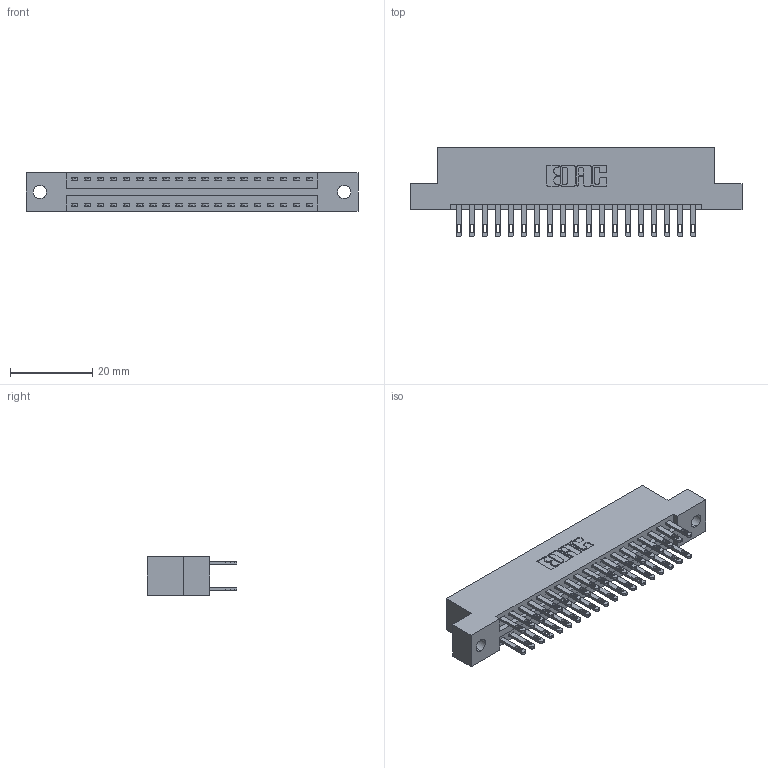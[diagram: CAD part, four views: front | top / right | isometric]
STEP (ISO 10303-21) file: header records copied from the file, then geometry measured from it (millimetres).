
FILE_DESCRIPTION (( 'STEP AP203' ), '1' );
FILE_NAME ('896-038-500-202.STEP', '2021-07-27T20:37:14', ( '' ), ( '' ), 'SwSTEP 2.0', 'SolidWorks 2020', '' );
FILE_SCHEMA (( 'CONFIG_CONTROL_DESIGN' ));
Length unit declared in the file: inch
Products named in the file (3): 896-038-500-202; 846 Part_Flush Mounting Lugs - 0.128 Dia; 345-292-001_345-293-100
Assembly tree (39 placements, depth 2):
  896-038-500-202
    846 Part_Flush Mounting Lugs - 0.128 Dia
    345-292-001_345-293-100  x38
Bounding box: 80.9 x 21.84 x 9.4 mm (x, y, z)
Volume: 7789.5 mm3; surface area: 10474.1 mm2
Topology: 39 solids, 39 shells, 1946 faces, 5915 edges, 3942 vertices
Faces by surface type: plane 1178, cylinder 768
Entity records: 15429 total; most frequent: CARTESIAN_POINT 2572, ORIENTED_EDGE 2506, DIRECTION 2321, EDGE_CURVE 1253, LINE 1041, VECTOR 1041, VERTEX_POINT 834, AXIS2_PLACEMENT_3D 640
